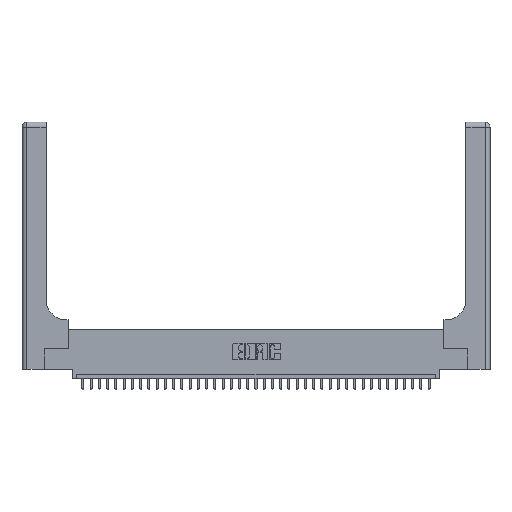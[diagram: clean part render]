
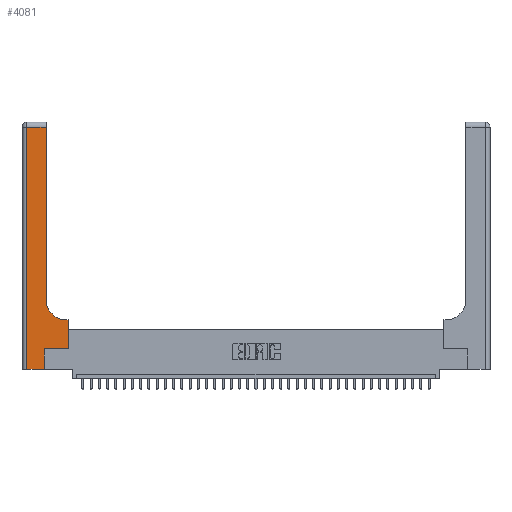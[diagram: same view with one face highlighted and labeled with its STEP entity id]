
A CAD part, top view. The second image highlights one B-rep face of the part: STEP entity #4081.
In plain terms, the highlighted planar face has unit normal (0, 0, 1).
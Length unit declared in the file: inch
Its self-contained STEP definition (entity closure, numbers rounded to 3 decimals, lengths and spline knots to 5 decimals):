
#32 = EDGE_CURVE ( 'NONE', #19004, #25727, #17016, .T. ) ;
#259 = VERTEX_POINT ( 'NONE', #14345 ) ;
#422 = DIRECTION ( 'NONE',  ( -1., 0., 0. ) ) ;
#1541 = EDGE_CURVE ( 'NONE', #25727, #24855, #30539, .T. ) ;
#3078 = EDGE_LOOP ( 'NONE', ( #17889, #23444, #11388, #15210, #27492, #13630, #22940, #21635, #33505 ) ) ;
#3211 = CARTESIAN_POINT ( 'NONE',  ( 0.5585, 0.25, 0.37 ) ) ;
#3420 = VERTEX_POINT ( 'NONE', #22783 ) ;
#3798 = EDGE_CURVE ( 'NONE', #24855, #259, #26303, .T. ) ;
#4081 = ADVANCED_FACE ( 'NONE', ( #4633 ), #20763, .F. ) ;
#4633 = FACE_OUTER_BOUND ( 'NONE', #3078, .T. ) ;
#5187 = DIRECTION ( 'NONE',  ( 1., 0., 0. ) ) ;
#6002 = VECTOR ( 'NONE', #17510, 39.37008 ) ;
#7406 = CARTESIAN_POINT ( 'NONE',  ( 0.269, 0., 0.37 ) ) ;
#7978 = CARTESIAN_POINT ( 'NONE',  ( 0., 2.94, 0.37 ) ) ;
#9690 = VECTOR ( 'NONE', #22450, 39.37008 ) ;
#9914 = EDGE_CURVE ( 'NONE', #3420, #12551, #34053, .T. ) ;
#10416 = DIRECTION ( 'NONE',  ( 1., 0., 0. ) ) ;
#11371 = EDGE_CURVE ( 'NONE', #12551, #20600, #12589, .T. ) ;
#11388 = ORIENTED_EDGE ( 'NONE', *, *, #26882, .T. ) ;
#12195 = AXIS2_PLACEMENT_3D ( 'NONE', #27945, #19679, #5187 ) ;
#12495 = CARTESIAN_POINT ( 'NONE',  ( 0.269, 0.25, 0.37 ) ) ;
#12551 = VERTEX_POINT ( 'NONE', #13711 ) ;
#12589 = CIRCLE ( 'NONE', #12195, 0.25 ) ;
#13223 = LINE ( 'NONE', #34895, #6002 ) ;
#13630 = ORIENTED_EDGE ( 'NONE', *, *, #3798, .T. ) ;
#13711 = CARTESIAN_POINT ( 'NONE',  ( 0.5415, 0.6, 0.37 ) ) ;
#14345 = CARTESIAN_POINT ( 'NONE',  ( 0.5585, 0.25, 0.37 ) ) ;
#15210 = ORIENTED_EDGE ( 'NONE', *, *, #32, .T. ) ;
#15554 = VECTOR ( 'NONE', #19918, 39.37008 ) ;
#15649 = DIRECTION ( 'NONE',  ( -1., 0., 0. ) ) ;
#17016 = LINE ( 'NONE', #37246, #32412 ) ;
#17048 = CARTESIAN_POINT ( 'NONE',  ( 0.269, 0., 0.37 ) ) ;
#17339 = LINE ( 'NONE', #7978, #9690 ) ;
#17510 = DIRECTION ( 'NONE',  ( 0., -1., 0. ) ) ;
#17889 = ORIENTED_EDGE ( 'NONE', *, *, #31916, .T. ) ;
#17953 = CARTESIAN_POINT ( 'NONE',  ( 0.06, 0., 0.37 ) ) ;
#18547 = VECTOR ( 'NONE', #422, 39.37008 ) ;
#19004 = VERTEX_POINT ( 'NONE', #17953 ) ;
#19679 = DIRECTION ( 'NONE',  ( 0., 0., -1. ) ) ;
#19918 = DIRECTION ( 'NONE',  ( 0., 1., 0. ) ) ;
#20600 = VERTEX_POINT ( 'NONE', #21745 ) ;
#20763 = PLANE ( 'NONE',  #30766 ) ;
#21635 = ORIENTED_EDGE ( 'NONE', *, *, #9914, .T. ) ;
#21745 = CARTESIAN_POINT ( 'NONE',  ( 0.2915, 0.85, 0.37 ) ) ;
#22450 = DIRECTION ( 'NONE',  ( -1., 0., 0. ) ) ;
#22783 = CARTESIAN_POINT ( 'NONE',  ( 0.5585, 0.6, 0.37 ) ) ;
#22940 = ORIENTED_EDGE ( 'NONE', *, *, #23788, .T. ) ;
#23444 = ORIENTED_EDGE ( 'NONE', *, *, #35139, .T. ) ;
#23788 = EDGE_CURVE ( 'NONE', #259, #3420, #27017, .T. ) ;
#23812 = VECTOR ( 'NONE', #24002, 39.37008 ) ;
#24002 = DIRECTION ( 'NONE',  ( 0., 1., 0. ) ) ;
#24855 = VERTEX_POINT ( 'NONE', #12495 ) ;
#25271 = VERTEX_POINT ( 'NONE', #31194 ) ;
#25727 = VERTEX_POINT ( 'NONE', #7406 ) ;
#26303 = LINE ( 'NONE', #31636, #27200 ) ;
#26737 = CARTESIAN_POINT ( 'NONE',  ( 0.2915, 3., 0.37 ) ) ;
#26882 = EDGE_CURVE ( 'NONE', #25271, #19004, #13223, .T. ) ;
#27017 = LINE ( 'NONE', #3211, #23812 ) ;
#27200 = VECTOR ( 'NONE', #28584, 39.37008 ) ;
#27492 = ORIENTED_EDGE ( 'NONE', *, *, #1541, .T. ) ;
#27945 = CARTESIAN_POINT ( 'NONE',  ( 0.5415, 0.85, 0.37 ) ) ;
#28584 = DIRECTION ( 'NONE',  ( 1., 0., 0. ) ) ;
#28877 = VERTEX_POINT ( 'NONE', #28974 ) ;
#28916 = CARTESIAN_POINT ( 'NONE',  ( 0.2915, 0.6, 0.37 ) ) ;
#28974 = CARTESIAN_POINT ( 'NONE',  ( 0.2915, 2.94, 0.37 ) ) ;
#29339 = VECTOR ( 'NONE', #32486, 39.37008 ) ;
#29935 = DIRECTION ( 'NONE',  ( 0., 0., -1. ) ) ;
#30539 = LINE ( 'NONE', #17048, #15554 ) ;
#30766 = AXIS2_PLACEMENT_3D ( 'NONE', #36233, #29935, #15649 ) ;
#31194 = CARTESIAN_POINT ( 'NONE',  ( 0.06, 2.94, 0.37 ) ) ;
#31636 = CARTESIAN_POINT ( 'NONE',  ( 0.269, 0.25, 0.37 ) ) ;
#31916 = EDGE_CURVE ( 'NONE', #20600, #28877, #37180, .T. ) ;
#32412 = VECTOR ( 'NONE', #10416, 39.37008 ) ;
#32486 = DIRECTION ( 'NONE',  ( 0., 1., 0. ) ) ;
#33505 = ORIENTED_EDGE ( 'NONE', *, *, #11371, .T. ) ;
#34053 = LINE ( 'NONE', #28916, #18547 ) ;
#34895 = CARTESIAN_POINT ( 'NONE',  ( 0.06, 3., 0.37 ) ) ;
#35139 = EDGE_CURVE ( 'NONE', #28877, #25271, #17339, .T. ) ;
#36233 = CARTESIAN_POINT ( 'NONE',  ( 0., 3., 0.37 ) ) ;
#37180 = LINE ( 'NONE', #26737, #29339 ) ;
#37246 = CARTESIAN_POINT ( 'NONE',  ( 0., 0., 0.37 ) ) ;
